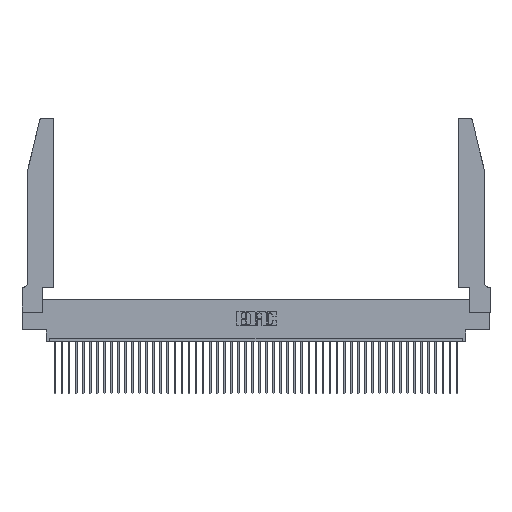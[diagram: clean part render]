
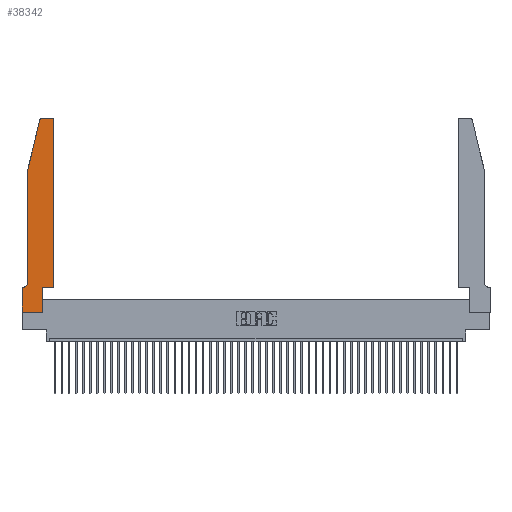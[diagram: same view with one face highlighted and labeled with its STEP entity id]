
A CAD part, top view. The second image highlights one B-rep face of the part: STEP entity #38342.
In plain terms, the highlighted planar face has unit normal (0, 0, 1).
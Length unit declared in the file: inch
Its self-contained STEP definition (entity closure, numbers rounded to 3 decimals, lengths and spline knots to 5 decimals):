
#261 = VERTEX_POINT ( 'NONE', #18640 ) ;
#490 = VERTEX_POINT ( 'NONE', #5487 ) ;
#744 = LINE ( 'NONE', #31584, #26646 ) ;
#930 = CARTESIAN_POINT ( 'NONE',  ( 0.0055, 0.42, 0.37 ) ) ;
#940 = EDGE_CURVE ( 'NONE', #14594, #13685, #42928, .T. ) ;
#1735 = CARTESIAN_POINT ( 'NONE',  ( 0., 0., 0.37 ) ) ;
#1961 = CARTESIAN_POINT ( 'NONE',  ( 0., 0.35, 0.37 ) ) ;
#2032 = ORIENTED_EDGE ( 'NONE', *, *, #6817, .T. ) ;
#2744 = CIRCLE ( 'NONE', #9024, 0.03 ) ;
#2925 = ORIENTED_EDGE ( 'NONE', *, *, #21486, .T. ) ;
#3063 = DIRECTION ( 'NONE',  ( 1., 0., 0. ) ) ;
#3733 = EDGE_CURVE ( 'NONE', #490, #28729, #28701, .T. ) ;
#4075 = LINE ( 'NONE', #11860, #34849 ) ;
#4760 = DIRECTION ( 'NONE',  ( 0., 1., 0. ) ) ;
#4940 = DIRECTION ( 'NONE',  ( 1., 0., 0. ) ) ;
#5069 = CARTESIAN_POINT ( 'NONE',  ( 0.25487, 2.72718, 0.37 ) ) ;
#5487 = CARTESIAN_POINT ( 'NONE',  ( 0.0755, 0.42, 0.37 ) ) ;
#6641 = ORIENTED_EDGE ( 'NONE', *, *, #940, .T. ) ;
#6817 = EDGE_CURVE ( 'NONE', #28729, #31119, #8858, .T. ) ;
#8082 = DIRECTION ( 'NONE',  ( -1., 0., 0. ) ) ;
#8157 = ORIENTED_EDGE ( 'NONE', *, *, #18838, .T. ) ;
#8858 = LINE ( 'NONE', #43372, #21722 ) ;
#9024 = AXIS2_PLACEMENT_3D ( 'NONE', #9374, #10175, #3063 ) ;
#9374 = CARTESIAN_POINT ( 'NONE',  ( 0.284, 2.72, 0.37 ) ) ;
#9659 = VERTEX_POINT ( 'NONE', #45461 ) ;
#9866 = EDGE_CURVE ( 'NONE', #11778, #9659, #4075, .T. ) ;
#10175 = DIRECTION ( 'NONE',  ( 0., 0., 1. ) ) ;
#11407 = VERTEX_POINT ( 'NONE', #17826 ) ;
#11615 = CARTESIAN_POINT ( 'NONE',  ( 0.4505, 0.35, 0.37 ) ) ;
#11778 = VERTEX_POINT ( 'NONE', #1735 ) ;
#11860 = CARTESIAN_POINT ( 'NONE',  ( 0., 0., 0.37 ) ) ;
#13626 = EDGE_LOOP ( 'NONE', ( #8157, #23790, #6641, #41172, #39438, #2032, #39035, #17656, #28322, #14653, #24351, #2925 ) ) ;
#13685 = VERTEX_POINT ( 'NONE', #17119 ) ;
#13749 = DIRECTION ( 'NONE',  ( 0., -1., 0. ) ) ;
#13760 = CARTESIAN_POINT ( 'NONE',  ( 0., 0.35, 0.37 ) ) ;
#14304 = LINE ( 'NONE', #26188, #22645 ) ;
#14594 = VERTEX_POINT ( 'NONE', #5069 ) ;
#14653 = ORIENTED_EDGE ( 'NONE', *, *, #38481, .T. ) ;
#14741 = EDGE_CURVE ( 'NONE', #13685, #490, #43770, .T. ) ;
#15628 = DIRECTION ( 'NONE',  ( 0., -1., 0. ) ) ;
#15955 = CARTESIAN_POINT ( 'NONE',  ( 0., 0., 0.37 ) ) ;
#16074 = VECTOR ( 'NONE', #15628, 39.37008 ) ;
#17119 = CARTESIAN_POINT ( 'NONE',  ( 0.0755, 2., 0.37 ) ) ;
#17156 = CARTESIAN_POINT ( 'NONE',  ( 0.0755, 2., 0.37 ) ) ;
#17294 = EDGE_CURVE ( 'NONE', #32973, #14594, #2744, .T. ) ;
#17656 = ORIENTED_EDGE ( 'NONE', *, *, #9866, .T. ) ;
#17826 = CARTESIAN_POINT ( 'NONE',  ( 0.4505, 2.72, 0.37 ) ) ;
#18640 = CARTESIAN_POINT ( 'NONE',  ( 0.2865, 0.35, 0.37 ) ) ;
#18838 = EDGE_CURVE ( 'NONE', #34875, #32973, #744, .T. ) ;
#19195 = DIRECTION ( 'NONE',  ( 0., 0., -1. ) ) ;
#19226 = VERTEX_POINT ( 'NONE', #11615 ) ;
#20938 = DIRECTION ( 'NONE',  ( 0., 0., 1. ) ) ;
#21238 = DIRECTION ( 'NONE',  ( 1., 0., 0. ) ) ;
#21486 = EDGE_CURVE ( 'NONE', #11407, #34875, #26897, .T. ) ;
#21564 = VECTOR ( 'NONE', #33837, 39.37008 ) ;
#21722 = VECTOR ( 'NONE', #8082, 39.37008 ) ;
#22081 = CARTESIAN_POINT ( 'NONE',  ( 0.4205, 2.75, 0.37 ) ) ;
#22269 = AXIS2_PLACEMENT_3D ( 'NONE', #22597, #26365, #4940 ) ;
#22275 = DIRECTION ( 'NONE',  ( -0.239, -0.971, 0. ) ) ;
#22478 = AXIS2_PLACEMENT_3D ( 'NONE', #930, #19195, #44662 ) ;
#22597 = CARTESIAN_POINT ( 'NONE',  ( 0.4205, 2.72, 0.37 ) ) ;
#22645 = VECTOR ( 'NONE', #4760, 39.37008 ) ;
#23790 = ORIENTED_EDGE ( 'NONE', *, *, #17294, .T. ) ;
#24351 = ORIENTED_EDGE ( 'NONE', *, *, #44798, .T. ) ;
#25589 = LINE ( 'NONE', #15955, #16074 ) ;
#26188 = CARTESIAN_POINT ( 'NONE',  ( 0.4505, 0.35, 0.37 ) ) ;
#26365 = DIRECTION ( 'NONE',  ( 0., 0., 1. ) ) ;
#26646 = VECTOR ( 'NONE', #28495, 39.37008 ) ;
#26897 = CIRCLE ( 'NONE', #22269, 0.03 ) ;
#27345 = VECTOR ( 'NONE', #22275, 39.37008 ) ;
#28322 = ORIENTED_EDGE ( 'NONE', *, *, #44845, .T. ) ;
#28495 = DIRECTION ( 'NONE',  ( -1., 0., 0. ) ) ;
#28701 = CIRCLE ( 'NONE', #22478, 0.07 ) ;
#28729 = VERTEX_POINT ( 'NONE', #39565 ) ;
#30408 = VECTOR ( 'NONE', #13749, 39.37008 ) ;
#31119 = VERTEX_POINT ( 'NONE', #1961 ) ;
#31581 = LINE ( 'NONE', #40829, #21564 ) ;
#31584 = CARTESIAN_POINT ( 'NONE',  ( 0.2605, 2.75, 0.37 ) ) ;
#32973 = VERTEX_POINT ( 'NONE', #41584 ) ;
#33328 = CARTESIAN_POINT ( 'NONE',  ( 0.4505, 0.35, 0.37 ) ) ;
#33837 = DIRECTION ( 'NONE',  ( 0., 1., 0. ) ) ;
#34849 = VECTOR ( 'NONE', #45357, 39.37008 ) ;
#34875 = VERTEX_POINT ( 'NONE', #22081 ) ;
#37148 = LINE ( 'NONE', #33328, #37758 ) ;
#37758 = VECTOR ( 'NONE', #44261, 39.37008 ) ;
#38342 = ADVANCED_FACE ( 'NONE', ( #44473 ), #46080, .T. ) ;
#38481 = EDGE_CURVE ( 'NONE', #261, #19226, #37148, .T. ) ;
#39035 = ORIENTED_EDGE ( 'NONE', *, *, #43493, .T. ) ;
#39438 = ORIENTED_EDGE ( 'NONE', *, *, #3733, .T. ) ;
#39565 = CARTESIAN_POINT ( 'NONE',  ( 0.0055, 0.35, 0.37 ) ) ;
#40829 = CARTESIAN_POINT ( 'NONE',  ( 0.2865, 0.35, 0.37 ) ) ;
#41172 = ORIENTED_EDGE ( 'NONE', *, *, #14741, .T. ) ;
#41584 = CARTESIAN_POINT ( 'NONE',  ( 0.284, 2.75, 0.37 ) ) ;
#42928 = LINE ( 'NONE', #43793, #27345 ) ;
#43023 = AXIS2_PLACEMENT_3D ( 'NONE', #13760, #20938, #21238 ) ;
#43372 = CARTESIAN_POINT ( 'NONE',  ( 0.0755, 0.35, 0.37 ) ) ;
#43493 = EDGE_CURVE ( 'NONE', #31119, #11778, #25589, .T. ) ;
#43770 = LINE ( 'NONE', #17156, #30408 ) ;
#43793 = CARTESIAN_POINT ( 'NONE',  ( 0.0755, 2., 0.37 ) ) ;
#44261 = DIRECTION ( 'NONE',  ( 1., 0., 0. ) ) ;
#44473 = FACE_OUTER_BOUND ( 'NONE', #13626, .T. ) ;
#44662 = DIRECTION ( 'NONE',  ( -1., 0., 0. ) ) ;
#44798 = EDGE_CURVE ( 'NONE', #19226, #11407, #14304, .T. ) ;
#44845 = EDGE_CURVE ( 'NONE', #9659, #261, #31581, .T. ) ;
#45357 = DIRECTION ( 'NONE',  ( 1., 0., 0. ) ) ;
#45461 = CARTESIAN_POINT ( 'NONE',  ( 0.2865, 0., 0.37 ) ) ;
#46080 = PLANE ( 'NONE',  #43023 ) ;
